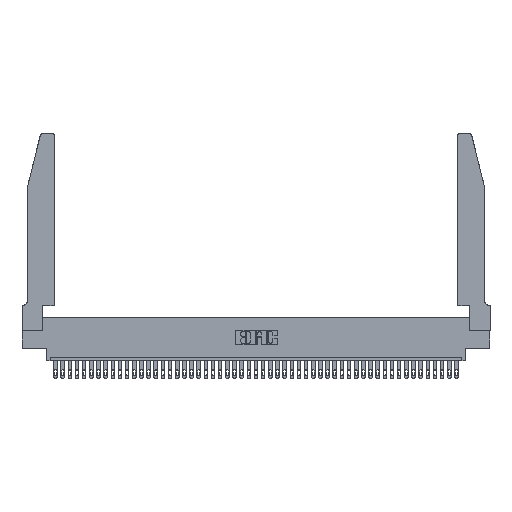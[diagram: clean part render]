
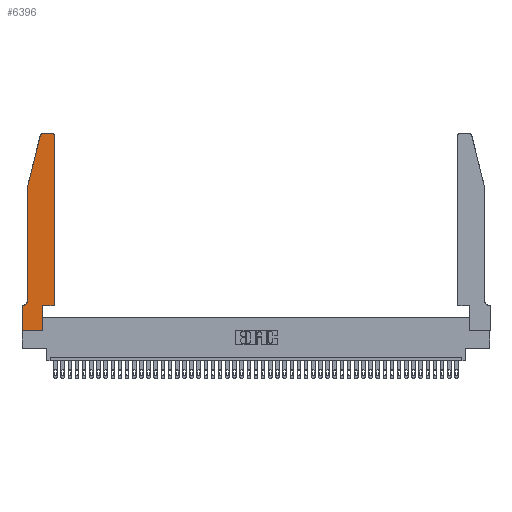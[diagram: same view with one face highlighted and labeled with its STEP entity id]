
A CAD part, top view. The second image highlights one B-rep face of the part: STEP entity #6396.
In plain terms, the highlighted planar face has unit normal (0, 0, 1).
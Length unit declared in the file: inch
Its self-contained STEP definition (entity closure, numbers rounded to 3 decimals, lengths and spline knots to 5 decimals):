
#199 = AXIS2_PLACEMENT_3D ( 'NONE', #29037, #11217, #39363 ) ;
#236 = ORIENTED_EDGE ( 'NONE', *, *, #38454, .T. ) ;
#1111 = ORIENTED_EDGE ( 'NONE', *, *, #9170, .T. ) ;
#1484 = DIRECTION ( 'NONE',  ( -0.239, -0.971, 0. ) ) ;
#2596 = VERTEX_POINT ( 'NONE', #45654 ) ;
#3042 = CIRCLE ( 'NONE', #199, 0.07 ) ;
#3398 = LINE ( 'NONE', #21448, #10588 ) ;
#3625 = DIRECTION ( 'NONE',  ( 1., 0., 0. ) ) ;
#3949 = AXIS2_PLACEMENT_3D ( 'NONE', #13635, #24531, #6972 ) ;
#4420 = ORIENTED_EDGE ( 'NONE', *, *, #23177, .T. ) ;
#6396 = ADVANCED_FACE ( 'NONE', ( #16519 ), #31492, .T. ) ;
#6428 = VECTOR ( 'NONE', #15560, 39.37008 ) ;
#6800 = CARTESIAN_POINT ( 'NONE',  ( 0., 0., 0.37 ) ) ;
#6930 = DIRECTION ( 'NONE',  ( 0., -1., 0. ) ) ;
#6972 = DIRECTION ( 'NONE',  ( 1., 0., 0. ) ) ;
#7003 = VECTOR ( 'NONE', #10093, 39.37008 ) ;
#7342 = CARTESIAN_POINT ( 'NONE',  ( 0.4505, 0.35, 0.37 ) ) ;
#7358 = VECTOR ( 'NONE', #15098, 39.37008 ) ;
#7461 = ORIENTED_EDGE ( 'NONE', *, *, #30590, .T. ) ;
#7715 = DIRECTION ( 'NONE',  ( 0., 1., 0. ) ) ;
#7822 = VECTOR ( 'NONE', #44748, 39.37008 ) ;
#8308 = ORIENTED_EDGE ( 'NONE', *, *, #14280, .T. ) ;
#8762 = VERTEX_POINT ( 'NONE', #42047 ) ;
#8913 = ORIENTED_EDGE ( 'NONE', *, *, #26092, .T. ) ;
#9170 = EDGE_CURVE ( 'NONE', #19988, #16704, #38813, .T. ) ;
#9282 = CARTESIAN_POINT ( 'NONE',  ( 0.4205, 2.72, 0.37 ) ) ;
#10093 = DIRECTION ( 'NONE',  ( 1., 0., 0. ) ) ;
#10588 = VECTOR ( 'NONE', #7715, 39.37008 ) ;
#10803 = EDGE_CURVE ( 'NONE', #16704, #16754, #38569, .T. ) ;
#10864 = CARTESIAN_POINT ( 'NONE',  ( 0.0755, 0.35, 0.37 ) ) ;
#11217 = DIRECTION ( 'NONE',  ( 0., 0., -1. ) ) ;
#12570 = LINE ( 'NONE', #26150, #6428 ) ;
#13332 = VERTEX_POINT ( 'NONE', #33565 ) ;
#13635 = CARTESIAN_POINT ( 'NONE',  ( 0., 0.35, 0.37 ) ) ;
#14280 = EDGE_CURVE ( 'NONE', #8762, #43607, #15308, .T. ) ;
#14418 = DIRECTION ( 'NONE',  ( -1., 0., 0. ) ) ;
#15098 = DIRECTION ( 'NONE',  ( 0., 1., 0. ) ) ;
#15304 = EDGE_CURVE ( 'NONE', #44141, #13332, #3042, .T. ) ;
#15308 = LINE ( 'NONE', #6800, #7003 ) ;
#15560 = DIRECTION ( 'NONE',  ( 1., 0., 0. ) ) ;
#16047 = CARTESIAN_POINT ( 'NONE',  ( 0.4205, 2.75, 0.37 ) ) ;
#16519 = FACE_OUTER_BOUND ( 'NONE', #23602, .T. ) ;
#16684 = CARTESIAN_POINT ( 'NONE',  ( 0.2605, 2.75, 0.37 ) ) ;
#16704 = VERTEX_POINT ( 'NONE', #22936 ) ;
#16754 = VERTEX_POINT ( 'NONE', #16047 ) ;
#16904 = LINE ( 'NONE', #10864, #37300 ) ;
#17939 = CARTESIAN_POINT ( 'NONE',  ( 0.284, 2.72, 0.37 ) ) ;
#18200 = VERTEX_POINT ( 'NONE', #37165 ) ;
#18297 = LINE ( 'NONE', #30523, #36496 ) ;
#19549 = CARTESIAN_POINT ( 'NONE',  ( 0.0755, 2., 0.37 ) ) ;
#19988 = VERTEX_POINT ( 'NONE', #22286 ) ;
#21083 = AXIS2_PLACEMENT_3D ( 'NONE', #9282, #44563, #41440 ) ;
#21188 = DIRECTION ( 'NONE',  ( 0., 0., 1. ) ) ;
#21367 = ORIENTED_EDGE ( 'NONE', *, *, #30713, .T. ) ;
#21448 = CARTESIAN_POINT ( 'NONE',  ( 0.2865, 0.35, 0.37 ) ) ;
#21754 = VECTOR ( 'NONE', #1484, 39.37008 ) ;
#22286 = CARTESIAN_POINT ( 'NONE',  ( 0.4505, 0.35, 0.37 ) ) ;
#22605 = CARTESIAN_POINT ( 'NONE',  ( 0., 0.35, 0.37 ) ) ;
#22811 = CARTESIAN_POINT ( 'NONE',  ( 0., 0., 0.37 ) ) ;
#22936 = CARTESIAN_POINT ( 'NONE',  ( 0.4505, 2.72, 0.37 ) ) ;
#23177 = EDGE_CURVE ( 'NONE', #13332, #35323, #16904, .T. ) ;
#23588 = EDGE_CURVE ( 'NONE', #35323, #8762, #29522, .T. ) ;
#23602 = EDGE_LOOP ( 'NONE', ( #21367, #236, #32409, #7461, #44575, #4420, #36387, #8308, #8913, #24736, #1111, #43894 ) ) ;
#24369 = CARTESIAN_POINT ( 'NONE',  ( 0.284, 2.75, 0.37 ) ) ;
#24531 = DIRECTION ( 'NONE',  ( 0., 0., 1. ) ) ;
#24736 = ORIENTED_EDGE ( 'NONE', *, *, #42297, .T. ) ;
#26092 = EDGE_CURVE ( 'NONE', #43607, #18200, #3398, .T. ) ;
#26150 = CARTESIAN_POINT ( 'NONE',  ( 0.4505, 0.35, 0.37 ) ) ;
#26793 = AXIS2_PLACEMENT_3D ( 'NONE', #17939, #21188, #3625 ) ;
#29037 = CARTESIAN_POINT ( 'NONE',  ( 0.0055, 0.42, 0.37 ) ) ;
#29522 = LINE ( 'NONE', #22811, #44469 ) ;
#30523 = CARTESIAN_POINT ( 'NONE',  ( 0.0755, 2., 0.37 ) ) ;
#30590 = EDGE_CURVE ( 'NONE', #2596, #44141, #18297, .T. ) ;
#30713 = EDGE_CURVE ( 'NONE', #16754, #34504, #33742, .T. ) ;
#31492 = PLANE ( 'NONE',  #3949 ) ;
#32409 = ORIENTED_EDGE ( 'NONE', *, *, #37108, .T. ) ;
#33333 = LINE ( 'NONE', #19549, #21754 ) ;
#33565 = CARTESIAN_POINT ( 'NONE',  ( 0.0055, 0.35, 0.37 ) ) ;
#33742 = LINE ( 'NONE', #16684, #7822 ) ;
#34504 = VERTEX_POINT ( 'NONE', #24369 ) ;
#35323 = VERTEX_POINT ( 'NONE', #22605 ) ;
#35504 = CARTESIAN_POINT ( 'NONE',  ( 0.0755, 0.42, 0.37 ) ) ;
#36387 = ORIENTED_EDGE ( 'NONE', *, *, #23588, .T. ) ;
#36496 = VECTOR ( 'NONE', #41462, 39.37008 ) ;
#37108 = EDGE_CURVE ( 'NONE', #41813, #2596, #33333, .T. ) ;
#37165 = CARTESIAN_POINT ( 'NONE',  ( 0.2865, 0.35, 0.37 ) ) ;
#37300 = VECTOR ( 'NONE', #14418, 39.37008 ) ;
#38454 = EDGE_CURVE ( 'NONE', #34504, #41813, #39308, .T. ) ;
#38569 = CIRCLE ( 'NONE', #21083, 0.03 ) ;
#38813 = LINE ( 'NONE', #7342, #7358 ) ;
#39308 = CIRCLE ( 'NONE', #26793, 0.03 ) ;
#39363 = DIRECTION ( 'NONE',  ( -1., 0., 0. ) ) ;
#41302 = CARTESIAN_POINT ( 'NONE',  ( 0.25487, 2.72718, 0.37 ) ) ;
#41440 = DIRECTION ( 'NONE',  ( 1., 0., 0. ) ) ;
#41462 = DIRECTION ( 'NONE',  ( 0., -1., 0. ) ) ;
#41813 = VERTEX_POINT ( 'NONE', #41302 ) ;
#42047 = CARTESIAN_POINT ( 'NONE',  ( 0., 0., 0.37 ) ) ;
#42297 = EDGE_CURVE ( 'NONE', #18200, #19988, #12570, .T. ) ;
#43113 = CARTESIAN_POINT ( 'NONE',  ( 0.2865, 0., 0.37 ) ) ;
#43607 = VERTEX_POINT ( 'NONE', #43113 ) ;
#43894 = ORIENTED_EDGE ( 'NONE', *, *, #10803, .T. ) ;
#44141 = VERTEX_POINT ( 'NONE', #35504 ) ;
#44469 = VECTOR ( 'NONE', #6930, 39.37008 ) ;
#44563 = DIRECTION ( 'NONE',  ( 0., 0., 1. ) ) ;
#44575 = ORIENTED_EDGE ( 'NONE', *, *, #15304, .T. ) ;
#44748 = DIRECTION ( 'NONE',  ( -1., 0., 0. ) ) ;
#45654 = CARTESIAN_POINT ( 'NONE',  ( 0.0755, 2., 0.37 ) ) ;
